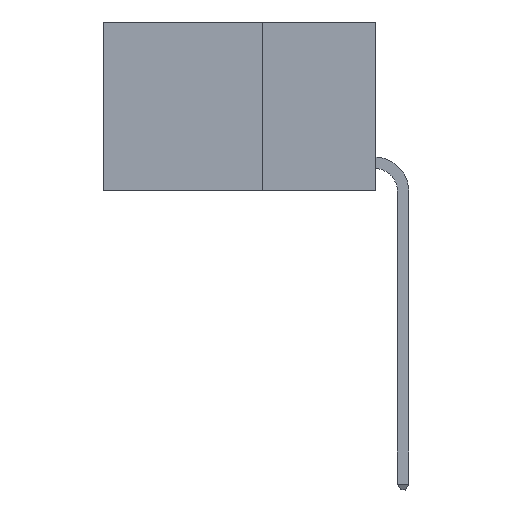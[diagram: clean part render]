
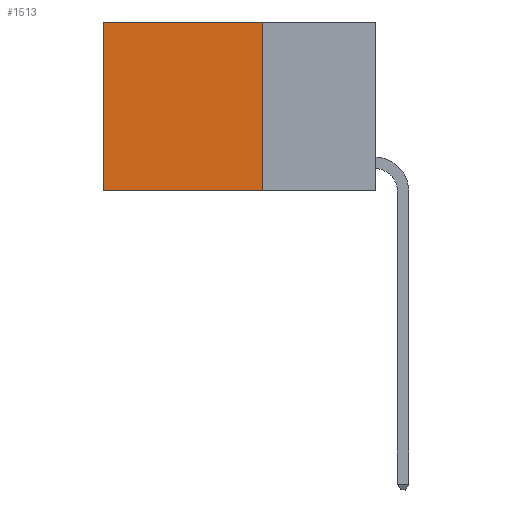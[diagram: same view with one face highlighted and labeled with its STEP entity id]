
A CAD part, left-side view. The second image highlights one B-rep face of the part: STEP entity #1513.
In plain terms, the highlighted planar face has unit normal (-1, 0, 0).
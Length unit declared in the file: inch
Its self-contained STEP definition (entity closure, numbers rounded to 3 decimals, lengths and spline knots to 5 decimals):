
#4 = DIRECTION ( 'NONE',  ( 0., 0., -1. ) ) ;
#367 = ORIENTED_EDGE ( 'NONE', *, *, #13598, .F. ) ;
#624 = EDGE_CURVE ( 'NONE', #20727, #13896, #27126, .T. ) ;
#695 = VECTOR ( 'NONE', #25599, 39.37008 ) ;
#1501 = ORIENTED_EDGE ( 'NONE', *, *, #27968, .F. ) ;
#1513 = ADVANCED_FACE ( 'NONE', ( #3884 ), #3721, .F. ) ;
#2958 = DIRECTION ( 'NONE',  ( 0., 0., -1. ) ) ;
#3721 = PLANE ( 'NONE',  #18971 ) ;
#3884 = FACE_OUTER_BOUND ( 'NONE', #22171, .T. ) ;
#4469 = CARTESIAN_POINT ( 'NONE',  ( 0.2625, 0.25, 0. ) ) ;
#5897 = EDGE_CURVE ( 'NONE', #13896, #21072, #26812, .T. ) ;
#7571 = ORIENTED_EDGE ( 'NONE', *, *, #624, .T. ) ;
#7771 = CARTESIAN_POINT ( 'NONE',  ( 0.2625, 0.25, -0.37 ) ) ;
#8146 = CARTESIAN_POINT ( 'NONE',  ( 0.2625, 0.25, 0. ) ) ;
#9757 = VECTOR ( 'NONE', #11660, 39.37008 ) ;
#10329 = DIRECTION ( 'NONE',  ( 0., 0., -1. ) ) ;
#11660 = DIRECTION ( 'NONE',  ( 0., 1., 0. ) ) ;
#12550 = CARTESIAN_POINT ( 'NONE',  ( 0.2625, 0.25, -0.37 ) ) ;
#13498 = VECTOR ( 'NONE', #4, 39.37008 ) ;
#13598 = EDGE_CURVE ( 'NONE', #20727, #16634, #21358, .T. ) ;
#13845 = CARTESIAN_POINT ( 'NONE',  ( 0.2625, 0.25, 0. ) ) ;
#13896 = VERTEX_POINT ( 'NONE', #27136 ) ;
#16634 = VERTEX_POINT ( 'NONE', #7771 ) ;
#18144 = LINE ( 'NONE', #12550, #695 ) ;
#18971 = AXIS2_PLACEMENT_3D ( 'NONE', #8146, #23318, #10329 ) ;
#20727 = VERTEX_POINT ( 'NONE', #21413 ) ;
#21072 = VERTEX_POINT ( 'NONE', #27024 ) ;
#21358 = LINE ( 'NONE', #4469, #13498 ) ;
#21413 = CARTESIAN_POINT ( 'NONE',  ( 0.2625, 0.25, 0. ) ) ;
#21687 = VECTOR ( 'NONE', #2958, 39.37008 ) ;
#22171 = EDGE_LOOP ( 'NONE', ( #26128, #1501, #367, #7571 ) ) ;
#23318 = DIRECTION ( 'NONE',  ( 1., 0., 0. ) ) ;
#24667 = CARTESIAN_POINT ( 'NONE',  ( 0.2625, 0.6, 0. ) ) ;
#25599 = DIRECTION ( 'NONE',  ( 0., 1., 0. ) ) ;
#26128 = ORIENTED_EDGE ( 'NONE', *, *, #5897, .T. ) ;
#26812 = LINE ( 'NONE', #24667, #21687 ) ;
#27024 = CARTESIAN_POINT ( 'NONE',  ( 0.2625, 0.6, -0.37 ) ) ;
#27126 = LINE ( 'NONE', #13845, #9757 ) ;
#27136 = CARTESIAN_POINT ( 'NONE',  ( 0.2625, 0.6, 0. ) ) ;
#27968 = EDGE_CURVE ( 'NONE', #16634, #21072, #18144, .T. ) ;
